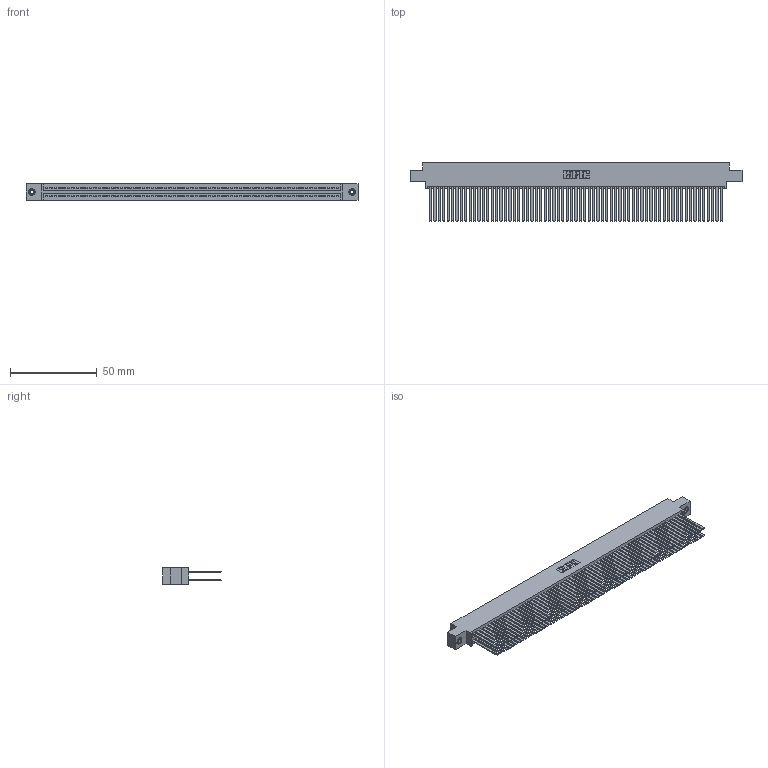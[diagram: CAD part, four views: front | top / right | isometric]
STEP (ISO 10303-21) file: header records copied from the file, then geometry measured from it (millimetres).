
FILE_DESCRIPTION (( 'STEP AP203' ), '1' );
FILE_NAME ('395-134-544-808.STEP', '2019-10-29T10:55:30', ( '' ), ( '' ), 'SwSTEP 2.0', 'SolidWorks 2016', '' );
FILE_SCHEMA (( 'CONFIG_CONTROL_DESIGN' ));
Length unit declared in the file: inch
Products named in the file (4): 345 Part_0.170 Offset - 0.156 Dia-TI; 345-292-001_345-293-144; 345-250-001_345-250-003-102; 395-134-544-808
Assembly tree (137 placements, depth 2):
  395-134-544-808
    345 Part_0.170 Offset - 0.156 Dia-TI
    345-292-001_345-293-144  x134
    345-250-001_345-250-003-102  x2
Bounding box: 191.39 x 33.96 x 9.4 mm (x, y, z)
Volume: 20582.3 mm3; surface area: 36570.7 mm2
Topology: 137 solids, 137 shells, 6086 faces, 18043 edges, 11842 vertices
Faces by surface type: plane 4002, cylinder 2068, cone 12, torus 4
Entity records: 50338 total; most frequent: CARTESIAN_POINT 8395, ORIENTED_EDGE 8322, DIRECTION 7395, EDGE_CURVE 4161, LINE 3745, VECTOR 3745, VERTEX_POINT 2768, AXIS2_PLACEMENT_3D 1825
